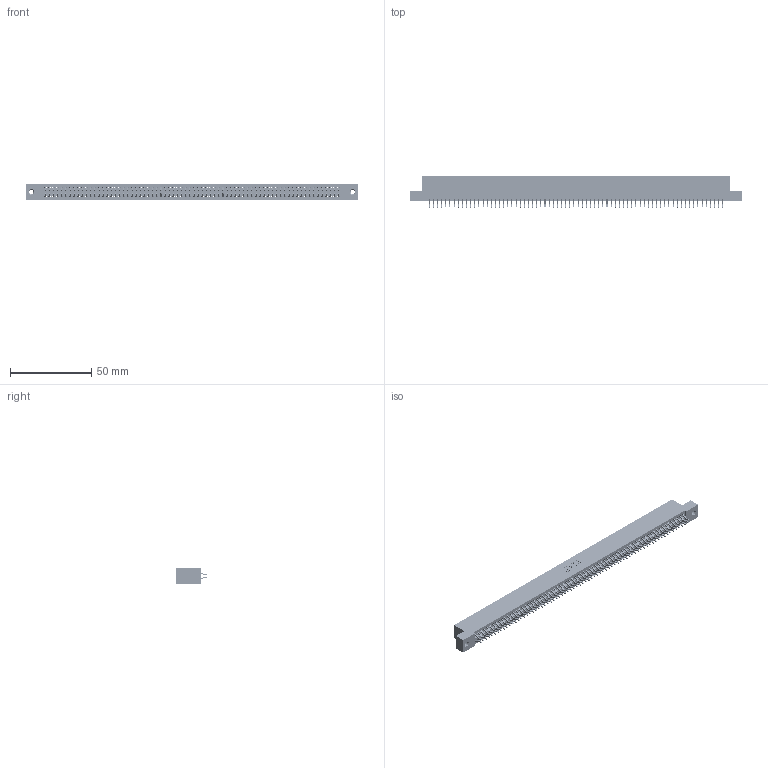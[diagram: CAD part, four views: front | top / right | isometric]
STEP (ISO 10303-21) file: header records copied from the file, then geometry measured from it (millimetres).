
FILE_DESCRIPTION (( 'STEP AP203' ), '1' );
FILE_NAME ('395-144-556-207.STEP', '2019-10-30T16:47:00', ( '' ), ( '' ), 'SwSTEP 2.0', 'SolidWorks 2016', '' );
FILE_SCHEMA (( 'CONFIG_CONTROL_DESIGN' ));
Length unit declared in the file: inch
Products named in the file (4): 345 Part_Flush Mounting Lugs - 0.156 Dia-TI; 345-292-001_556 Tail; 345-250-001_345-250-005-103; 395-144-556-207
Assembly tree (147 placements, depth 2):
  395-144-556-207
    345 Part_Flush Mounting Lugs - 0.156 Dia-TI
    345-292-001_556 Tail  x144
    345-250-001_345-250-005-103  x2
Bounding box: 204.09 x 19.24 x 9.4 mm (x, y, z)
Volume: 20084.7 mm3; surface area: 30171.4 mm2
Topology: 147 solids, 147 shells, 8250 faces, 24525 edges, 16150 vertices
Faces by surface type: plane 5440, cylinder 2794, cone 12, torus 4
Entity records: 53860 total; most frequent: CARTESIAN_POINT 8995, ORIENTED_EDGE 8910, DIRECTION 7909, EDGE_CURVE 4455, LINE 4007, VECTOR 4007, VERTEX_POINT 2964, AXIS2_PLACEMENT_3D 1951
